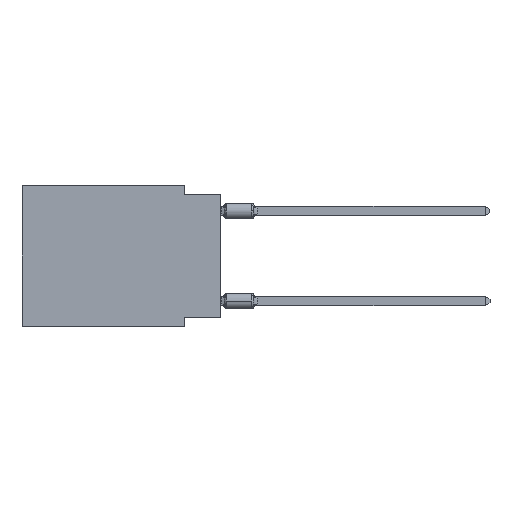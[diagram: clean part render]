
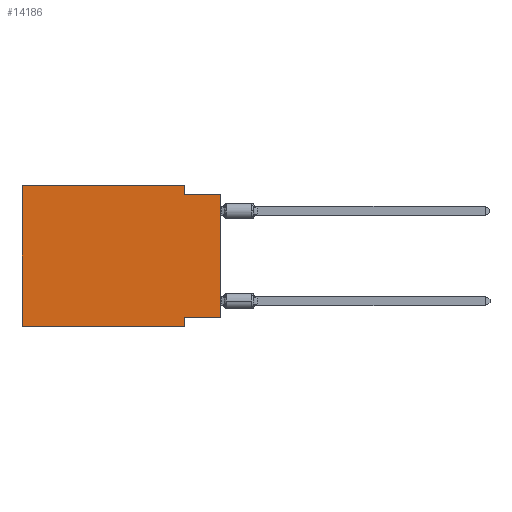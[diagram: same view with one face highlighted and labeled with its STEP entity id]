
A CAD part, left-side view. The second image highlights one B-rep face of the part: STEP entity #14186.
In plain terms, the highlighted planar face has unit normal (-1, 0, 0).
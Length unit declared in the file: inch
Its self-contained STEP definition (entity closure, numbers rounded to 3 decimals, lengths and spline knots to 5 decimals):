
#714 = CARTESIAN_POINT ( 'NONE',  ( 0., 0.1, -0.365 ) ) ;
#902 = LINE ( 'NONE', #17121, #3629 ) ;
#1935 = CARTESIAN_POINT ( 'NONE',  ( 0., 0.55, 0. ) ) ;
#1993 = CARTESIAN_POINT ( 'NONE',  ( 0., 0.1, 0. ) ) ;
#2427 = ORIENTED_EDGE ( 'NONE', *, *, #8465, .F. ) ;
#2605 = EDGE_CURVE ( 'NONE', #33369, #5071, #39147, .T. ) ;
#3629 = VECTOR ( 'NONE', #35662, 39.37008 ) ;
#4647 = CARTESIAN_POINT ( 'NONE',  ( 0., 0., -0.365 ) ) ;
#4792 = EDGE_CURVE ( 'NONE', #33369, #23122, #28267, .T. ) ;
#4894 = DIRECTION ( 'NONE',  ( 0., 1., 0. ) ) ;
#5071 = VERTEX_POINT ( 'NONE', #714 ) ;
#5613 = EDGE_CURVE ( 'NONE', #27419, #23122, #902, .T. ) ;
#5780 = DIRECTION ( 'NONE',  ( 0., 0., -1. ) ) ;
#6316 = ORIENTED_EDGE ( 'NONE', *, *, #45858, .T. ) ;
#7065 = LINE ( 'NONE', #7299, #31536 ) ;
#7125 = VECTOR ( 'NONE', #5780, 39.37008 ) ;
#7153 = EDGE_CURVE ( 'NONE', #5071, #42060, #37546, .T. ) ;
#7299 = CARTESIAN_POINT ( 'NONE',  ( 0., 0.55, 0. ) ) ;
#7784 = LINE ( 'NONE', #34281, #47480 ) ;
#7923 = CARTESIAN_POINT ( 'NONE',  ( 0., 0.55, 0. ) ) ;
#8465 = EDGE_CURVE ( 'NONE', #42020, #16417, #7065, .T. ) ;
#9776 = LINE ( 'NONE', #25012, #7125 ) ;
#10203 = VERTEX_POINT ( 'NONE', #23472 ) ;
#10884 = ORIENTED_EDGE ( 'NONE', *, *, #4792, .T. ) ;
#11937 = VECTOR ( 'NONE', #43038, 39.37008 ) ;
#14186 = ADVANCED_FACE ( 'NONE', ( #25447 ), #17429, .F. ) ;
#15010 = CARTESIAN_POINT ( 'NONE',  ( 0., 0.1, -0.39 ) ) ;
#15269 = DIRECTION ( 'NONE',  ( 0., -1., 0. ) ) ;
#15701 = ORIENTED_EDGE ( 'NONE', *, *, #2605, .F. ) ;
#16417 = VERTEX_POINT ( 'NONE', #1993 ) ;
#17121 = CARTESIAN_POINT ( 'NONE',  ( 0., 0., -0.025 ) ) ;
#17429 = PLANE ( 'NONE',  #45427 ) ;
#18208 = CARTESIAN_POINT ( 'NONE',  ( 0., 0., -0.025 ) ) ;
#18526 = DIRECTION ( 'NONE',  ( 0., -1., 0. ) ) ;
#18657 = CARTESIAN_POINT ( 'NONE',  ( 0., 0.1, -0.39 ) ) ;
#18878 = VECTOR ( 'NONE', #44791, 39.37008 ) ;
#20355 = ORIENTED_EDGE ( 'NONE', *, *, #7153, .F. ) ;
#20944 = DIRECTION ( 'NONE',  ( 1., 0., 0. ) ) ;
#21142 = CARTESIAN_POINT ( 'NONE',  ( 0., 0., -0.365 ) ) ;
#23122 = VERTEX_POINT ( 'NONE', #18208 ) ;
#23469 = CARTESIAN_POINT ( 'NONE',  ( 0., 0.1, -0.025 ) ) ;
#23472 = CARTESIAN_POINT ( 'NONE',  ( 0., 0.55, -0.39 ) ) ;
#25012 = CARTESIAN_POINT ( 'NONE',  ( 0., 0.1, 0. ) ) ;
#25447 = FACE_OUTER_BOUND ( 'NONE', #39760, .T. ) ;
#25877 = VECTOR ( 'NONE', #49210, 39.37008 ) ;
#27419 = VERTEX_POINT ( 'NONE', #23469 ) ;
#28267 = LINE ( 'NONE', #32768, #11937 ) ;
#28956 = DIRECTION ( 'NONE',  ( 0., 0., -1. ) ) ;
#31209 = CARTESIAN_POINT ( 'NONE',  ( 0., 0.55, 0. ) ) ;
#31536 = VECTOR ( 'NONE', #18526, 39.37008 ) ;
#31919 = VECTOR ( 'NONE', #4894, 39.37008 ) ;
#32415 = EDGE_CURVE ( 'NONE', #16417, #27419, #9776, .T. ) ;
#32768 = CARTESIAN_POINT ( 'NONE',  ( 0., 0., 0. ) ) ;
#33369 = VERTEX_POINT ( 'NONE', #21142 ) ;
#34281 = CARTESIAN_POINT ( 'NONE',  ( 0., 0.55, -0.39 ) ) ;
#35662 = DIRECTION ( 'NONE',  ( 0., -1., 0. ) ) ;
#37305 = EDGE_CURVE ( 'NONE', #10203, #42020, #38979, .T. ) ;
#37546 = LINE ( 'NONE', #15010, #18878 ) ;
#38979 = LINE ( 'NONE', #31209, #25877 ) ;
#39147 = LINE ( 'NONE', #4647, #31919 ) ;
#39760 = EDGE_LOOP ( 'NONE', ( #10884, #42091, #40702, #2427, #43851, #6316, #20355, #15701 ) ) ;
#40702 = ORIENTED_EDGE ( 'NONE', *, *, #32415, .F. ) ;
#42020 = VERTEX_POINT ( 'NONE', #7923 ) ;
#42060 = VERTEX_POINT ( 'NONE', #18657 ) ;
#42091 = ORIENTED_EDGE ( 'NONE', *, *, #5613, .F. ) ;
#43038 = DIRECTION ( 'NONE',  ( 0., 0., 1. ) ) ;
#43851 = ORIENTED_EDGE ( 'NONE', *, *, #37305, .F. ) ;
#44791 = DIRECTION ( 'NONE',  ( 0., 0., -1. ) ) ;
#45427 = AXIS2_PLACEMENT_3D ( 'NONE', #1935, #20944, #28956 ) ;
#45858 = EDGE_CURVE ( 'NONE', #10203, #42060, #7784, .T. ) ;
#47480 = VECTOR ( 'NONE', #15269, 39.37008 ) ;
#49210 = DIRECTION ( 'NONE',  ( 0., 0., 1. ) ) ;
